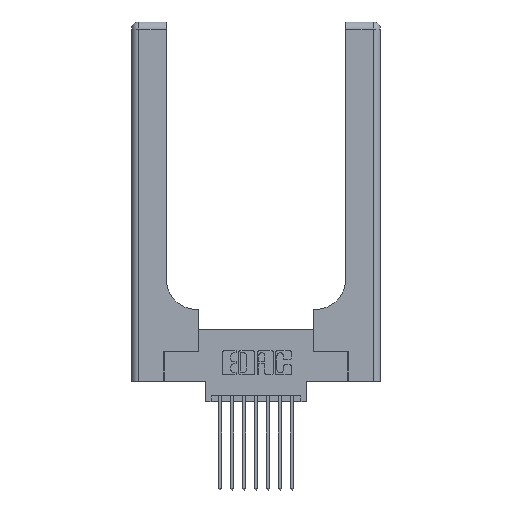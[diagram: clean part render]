
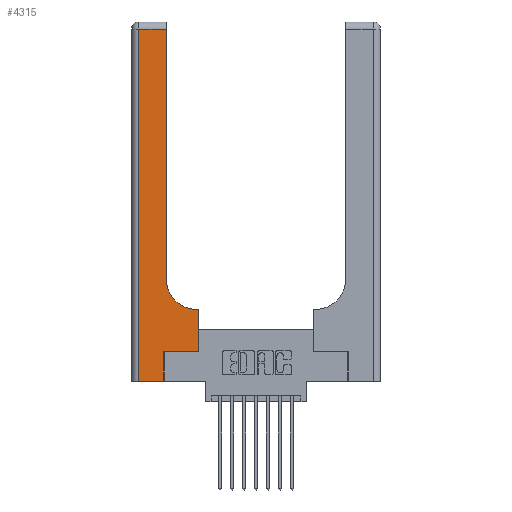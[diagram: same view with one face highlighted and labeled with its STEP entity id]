
A CAD part, top view. The second image highlights one B-rep face of the part: STEP entity #4315.
In plain terms, the highlighted planar face has unit normal (0, 0, 1).
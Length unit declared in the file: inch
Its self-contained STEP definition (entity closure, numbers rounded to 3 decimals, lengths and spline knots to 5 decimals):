
#1 = CARTESIAN_POINT ( 'NONE',  ( 0.2915, 0.6, 0.37 ) ) ;
#300 = LINE ( 'NONE', #1, #6388 ) ;
#656 = ORIENTED_EDGE ( 'NONE', *, *, #1291, .T. ) ;
#1101 = VECTOR ( 'NONE', #14720, 39.37008 ) ;
#1221 = ORIENTED_EDGE ( 'NONE', *, *, #2459, .T. ) ;
#1291 = EDGE_CURVE ( 'NONE', #10081, #11420, #7600, .T. ) ;
#1487 = VECTOR ( 'NONE', #10761, 39.37008 ) ;
#1702 = LINE ( 'NONE', #7164, #7381 ) ;
#2328 = CARTESIAN_POINT ( 'NONE',  ( 0.5585, 0.6, 0.37 ) ) ;
#2447 = VERTEX_POINT ( 'NONE', #2328 ) ;
#2459 = EDGE_CURVE ( 'NONE', #13523, #6411, #4707, .T. ) ;
#2547 = CARTESIAN_POINT ( 'NONE',  ( 0.269, 0., 0.37 ) ) ;
#2556 = ORIENTED_EDGE ( 'NONE', *, *, #14359, .T. ) ;
#2618 = EDGE_LOOP ( 'NONE', ( #656, #2556, #6151, #12897, #13266, #1221, #4838, #11615, #14770 ) ) ;
#2733 = EDGE_CURVE ( 'NONE', #2447, #7235, #300, .T. ) ;
#2857 = CARTESIAN_POINT ( 'NONE',  ( 0.2915, 0.85, 0.37 ) ) ;
#3544 = CARTESIAN_POINT ( 'NONE',  ( 0.269, 0.25, 0.37 ) ) ;
#3616 = DIRECTION ( 'NONE',  ( 0., 0., -1. ) ) ;
#3672 = DIRECTION ( 'NONE',  ( -1., 0., 0. ) ) ;
#3715 = PLANE ( 'NONE',  #10643 ) ;
#3846 = AXIS2_PLACEMENT_3D ( 'NONE', #10832, #3616, #12022 ) ;
#4315 = ADVANCED_FACE ( 'NONE', ( #15308 ), #3715, .F. ) ;
#4707 = LINE ( 'NONE', #3544, #1487 ) ;
#4717 = LINE ( 'NONE', #11138, #1101 ) ;
#4838 = ORIENTED_EDGE ( 'NONE', *, *, #9352, .T. ) ;
#4886 = DIRECTION ( 'NONE',  ( 0., 1., 0. ) ) ;
#4968 = VECTOR ( 'NONE', #14742, 39.37008 ) ;
#5417 = VERTEX_POINT ( 'NONE', #6451 ) ;
#5577 = CIRCLE ( 'NONE', #3846, 0.25 ) ;
#5772 = VECTOR ( 'NONE', #7922, 39.37008 ) ;
#6142 = DIRECTION ( 'NONE',  ( 0., 0., -1. ) ) ;
#6151 = ORIENTED_EDGE ( 'NONE', *, *, #7161, .T. ) ;
#6388 = VECTOR ( 'NONE', #3672, 39.37008 ) ;
#6411 = VERTEX_POINT ( 'NONE', #10710 ) ;
#6451 = CARTESIAN_POINT ( 'NONE',  ( 0.06, 2.94, 0.37 ) ) ;
#7161 = EDGE_CURVE ( 'NONE', #5417, #8625, #11734, .T. ) ;
#7164 = CARTESIAN_POINT ( 'NONE',  ( 0., 2.94, 0.37 ) ) ;
#7235 = VERTEX_POINT ( 'NONE', #10118 ) ;
#7381 = VECTOR ( 'NONE', #8382, 39.37008 ) ;
#7600 = LINE ( 'NONE', #9742, #13566 ) ;
#7922 = DIRECTION ( 'NONE',  ( 1., 0., 0. ) ) ;
#8382 = DIRECTION ( 'NONE',  ( -1., 0., 0. ) ) ;
#8587 = CARTESIAN_POINT ( 'NONE',  ( 0.5585, 0.25, 0.37 ) ) ;
#8625 = VERTEX_POINT ( 'NONE', #14139 ) ;
#8829 = VECTOR ( 'NONE', #4886, 39.37008 ) ;
#9352 = EDGE_CURVE ( 'NONE', #6411, #2447, #11977, .T. ) ;
#9626 = EDGE_CURVE ( 'NONE', #8625, #14522, #12170, .T. ) ;
#9742 = CARTESIAN_POINT ( 'NONE',  ( 0.2915, 3., 0.37 ) ) ;
#9820 = DIRECTION ( 'NONE',  ( 0., 1., 0. ) ) ;
#10081 = VERTEX_POINT ( 'NONE', #2857 ) ;
#10118 = CARTESIAN_POINT ( 'NONE',  ( 0.5415, 0.6, 0.37 ) ) ;
#10214 = CARTESIAN_POINT ( 'NONE',  ( 0.2915, 2.94, 0.37 ) ) ;
#10643 = AXIS2_PLACEMENT_3D ( 'NONE', #10929, #6142, #14510 ) ;
#10710 = CARTESIAN_POINT ( 'NONE',  ( 0.5585, 0.25, 0.37 ) ) ;
#10761 = DIRECTION ( 'NONE',  ( 1., 0., 0. ) ) ;
#10832 = CARTESIAN_POINT ( 'NONE',  ( 0.5415, 0.85, 0.37 ) ) ;
#10929 = CARTESIAN_POINT ( 'NONE',  ( 0., 3., 0.37 ) ) ;
#11138 = CARTESIAN_POINT ( 'NONE',  ( 0.269, 0., 0.37 ) ) ;
#11177 = EDGE_CURVE ( 'NONE', #7235, #10081, #5577, .T. ) ;
#11420 = VERTEX_POINT ( 'NONE', #10214 ) ;
#11615 = ORIENTED_EDGE ( 'NONE', *, *, #2733, .T. ) ;
#11734 = LINE ( 'NONE', #13547, #4968 ) ;
#11977 = LINE ( 'NONE', #8587, #8829 ) ;
#12022 = DIRECTION ( 'NONE',  ( 1., 0., 0. ) ) ;
#12170 = LINE ( 'NONE', #15032, #5772 ) ;
#12897 = ORIENTED_EDGE ( 'NONE', *, *, #9626, .T. ) ;
#13266 = ORIENTED_EDGE ( 'NONE', *, *, #14616, .T. ) ;
#13523 = VERTEX_POINT ( 'NONE', #13713 ) ;
#13547 = CARTESIAN_POINT ( 'NONE',  ( 0.06, 3., 0.37 ) ) ;
#13566 = VECTOR ( 'NONE', #9820, 39.37008 ) ;
#13713 = CARTESIAN_POINT ( 'NONE',  ( 0.269, 0.25, 0.37 ) ) ;
#14139 = CARTESIAN_POINT ( 'NONE',  ( 0.06, 0., 0.37 ) ) ;
#14359 = EDGE_CURVE ( 'NONE', #11420, #5417, #1702, .T. ) ;
#14510 = DIRECTION ( 'NONE',  ( -1., 0., 0. ) ) ;
#14522 = VERTEX_POINT ( 'NONE', #2547 ) ;
#14616 = EDGE_CURVE ( 'NONE', #14522, #13523, #4717, .T. ) ;
#14720 = DIRECTION ( 'NONE',  ( 0., 1., 0. ) ) ;
#14742 = DIRECTION ( 'NONE',  ( 0., -1., 0. ) ) ;
#14770 = ORIENTED_EDGE ( 'NONE', *, *, #11177, .T. ) ;
#15032 = CARTESIAN_POINT ( 'NONE',  ( 0., 0., 0.37 ) ) ;
#15308 = FACE_OUTER_BOUND ( 'NONE', #2618, .T. ) ;
